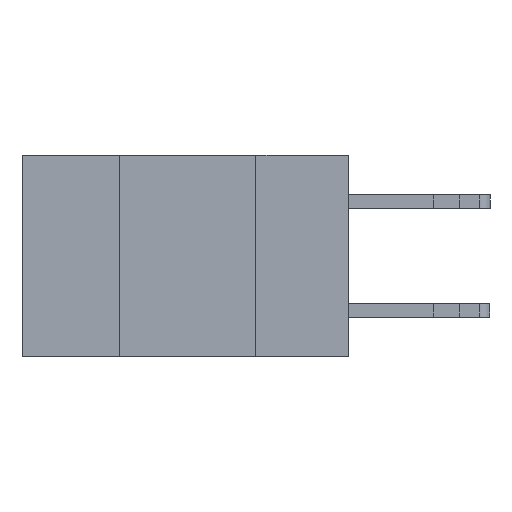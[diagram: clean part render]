
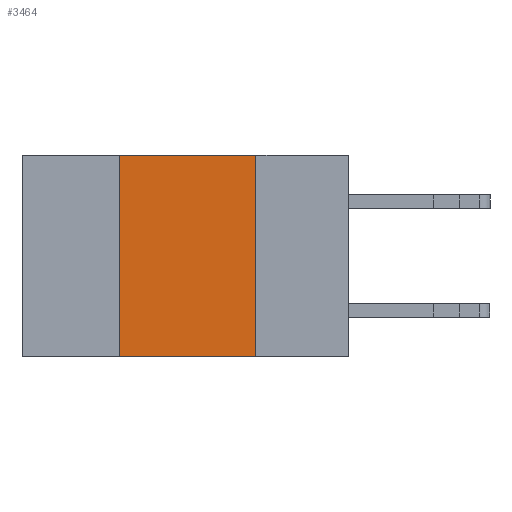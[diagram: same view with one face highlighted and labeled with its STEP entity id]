
A CAD part, left-side view. The second image highlights one B-rep face of the part: STEP entity #3464.
In plain terms, the highlighted planar face has unit normal (-1, 0, 0).
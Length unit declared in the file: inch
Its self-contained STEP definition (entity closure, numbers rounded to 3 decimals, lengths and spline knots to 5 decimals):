
#216 = CARTESIAN_POINT ( 'NONE',  ( 0., 0.6, -0.37 ) ) ;
#1620 = CARTESIAN_POINT ( 'NONE',  ( 0., 0.17, -0.37 ) ) ;
#1950 = PLANE ( 'NONE',  #2294 ) ;
#1984 = LINE ( 'NONE', #8965, #11886 ) ;
#2031 = DIRECTION ( 'NONE',  ( 0., 0., -1. ) ) ;
#2294 = AXIS2_PLACEMENT_3D ( 'NONE', #6222, #3637, #2031 ) ;
#2378 = LINE ( 'NONE', #5580, #8892 ) ;
#2404 = ORIENTED_EDGE ( 'NONE', *, *, #6097, .F. ) ;
#2666 = LINE ( 'NONE', #216, #15825 ) ;
#2916 = EDGE_CURVE ( 'NONE', #9856, #10223, #2666, .T. ) ;
#3308 = CARTESIAN_POINT ( 'NONE',  ( 0., 0.17, 0. ) ) ;
#3368 = DIRECTION ( 'NONE',  ( 0., 0., 1. ) ) ;
#3464 = ADVANCED_FACE ( 'NONE', ( #14629 ), #1950, .F. ) ;
#3637 = DIRECTION ( 'NONE',  ( 1., 0., 0. ) ) ;
#4030 = VECTOR ( 'NONE', #4633, 39.37008 ) ;
#4436 = LINE ( 'NONE', #3308, #4030 ) ;
#4633 = DIRECTION ( 'NONE',  ( 0., 0., -1. ) ) ;
#4979 = DIRECTION ( 'NONE',  ( 0., -1., 0. ) ) ;
#4996 = EDGE_CURVE ( 'NONE', #9625, #16117, #1984, .T. ) ;
#5580 = CARTESIAN_POINT ( 'NONE',  ( 0., 0.42, 0. ) ) ;
#6097 = EDGE_CURVE ( 'NONE', #9856, #9625, #2378, .T. ) ;
#6222 = CARTESIAN_POINT ( 'NONE',  ( 0., 0.6, 0. ) ) ;
#7685 = CARTESIAN_POINT ( 'NONE',  ( 0., 0.17, 0. ) ) ;
#8093 = ORIENTED_EDGE ( 'NONE', *, *, #14447, .F. ) ;
#8439 = EDGE_LOOP ( 'NONE', ( #8093, #11904, #2404, #9329 ) ) ;
#8892 = VECTOR ( 'NONE', #3368, 39.37008 ) ;
#8965 = CARTESIAN_POINT ( 'NONE',  ( 0., 0.6, 0. ) ) ;
#8983 = DIRECTION ( 'NONE',  ( 0., -1., 0. ) ) ;
#9310 = CARTESIAN_POINT ( 'NONE',  ( 0., 0.42, 0. ) ) ;
#9329 = ORIENTED_EDGE ( 'NONE', *, *, #2916, .T. ) ;
#9625 = VERTEX_POINT ( 'NONE', #9310 ) ;
#9856 = VERTEX_POINT ( 'NONE', #12266 ) ;
#10223 = VERTEX_POINT ( 'NONE', #1620 ) ;
#11886 = VECTOR ( 'NONE', #8983, 39.37008 ) ;
#11904 = ORIENTED_EDGE ( 'NONE', *, *, #4996, .F. ) ;
#12266 = CARTESIAN_POINT ( 'NONE',  ( 0., 0.42, -0.37 ) ) ;
#14447 = EDGE_CURVE ( 'NONE', #16117, #10223, #4436, .T. ) ;
#14629 = FACE_OUTER_BOUND ( 'NONE', #8439, .T. ) ;
#15825 = VECTOR ( 'NONE', #4979, 39.37008 ) ;
#16117 = VERTEX_POINT ( 'NONE', #7685 ) ;
